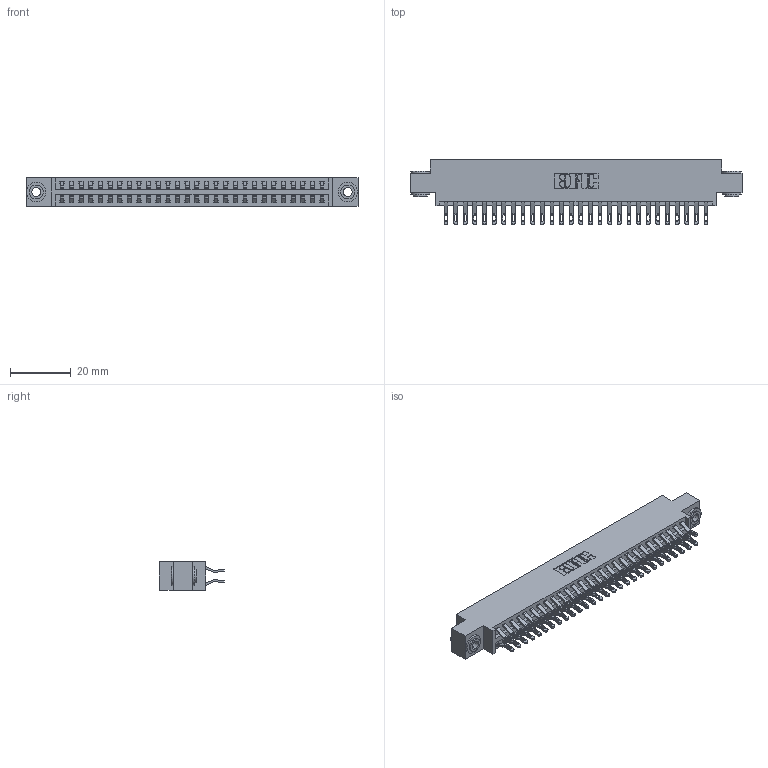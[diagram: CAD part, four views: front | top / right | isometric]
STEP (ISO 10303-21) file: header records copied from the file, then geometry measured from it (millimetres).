
FILE_DESCRIPTION (( 'STEP AP203' ), '1' );
FILE_NAME ('396-056-555-803.STEP', '2019-11-02T08:23:49', ( '' ), ( '' ), 'SwSTEP 2.0', 'SolidWorks 2016', '' );
FILE_SCHEMA (( 'CONFIG_CONTROL_DESIGN' ));
Length unit declared in the file: inch
Products named in the file (4): 345-250-002_345-250-002-102; 396-056-555-803; 346 Part_0.170 Offset - 0.156 Dia-TH; 345-292-001_555 Tail
Assembly tree (59 placements, depth 2):
  396-056-555-803
    346 Part_0.170 Offset - 0.156 Dia-TH
    345-292-001_555 Tail  x56
    345-250-002_345-250-002-102  x2
Bounding box: 109.47 x 21.46 x 9.4 mm (x, y, z)
Volume: 10593.6 mm3; surface area: 15314.3 mm2
Topology: 59 solids, 59 shells, 3412 faces, 10665 edges, 7106 vertices
Faces by surface type: plane 1938, cylinder 1466, cone 8
Entity records: 21266 total; most frequent: CARTESIAN_POINT 3537, ORIENTED_EDGE 3434, DIRECTION 3167, EDGE_CURVE 1717, LINE 1429, VECTOR 1429, VERTEX_POINT 1142, AXIS2_PLACEMENT_3D 869
